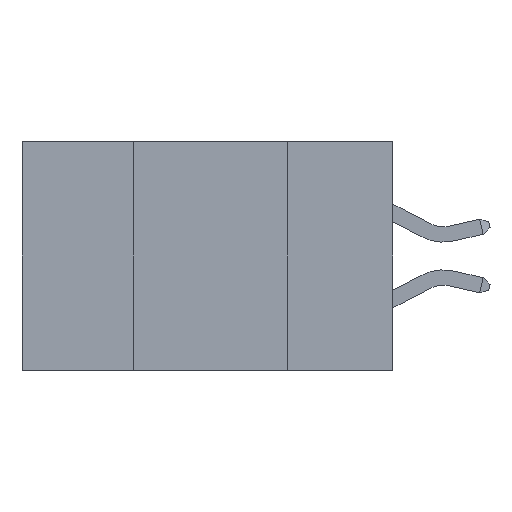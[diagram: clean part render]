
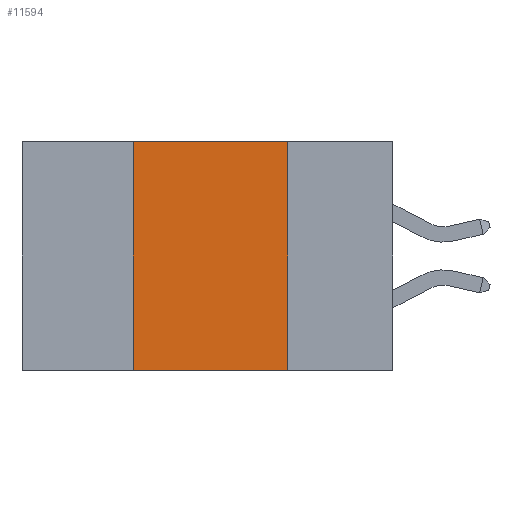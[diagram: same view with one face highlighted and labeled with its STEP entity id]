
A CAD part, left-side view. The second image highlights one B-rep face of the part: STEP entity #11594.
In plain terms, the highlighted planar face has unit normal (-1, 0, 0).
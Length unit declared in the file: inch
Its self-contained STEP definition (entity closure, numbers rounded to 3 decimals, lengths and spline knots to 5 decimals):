
#779 = CARTESIAN_POINT ( 'NONE',  ( 0., 0.6, -0.37 ) ) ;
#1283 = EDGE_CURVE ( 'NONE', #11097, #8057, #9412, .T. ) ;
#1348 = CARTESIAN_POINT ( 'NONE',  ( 0., 0.17, -0.37 ) ) ;
#2622 = DIRECTION ( 'NONE',  ( 0., -1., 0. ) ) ;
#2745 = CARTESIAN_POINT ( 'NONE',  ( 0., 0.6, 0. ) ) ;
#2826 = DIRECTION ( 'NONE',  ( 1., 0., 0. ) ) ;
#4833 = DIRECTION ( 'NONE',  ( 0., 0., 1. ) ) ;
#6314 = EDGE_CURVE ( 'NONE', #17043, #8785, #16749, .T. ) ;
#8057 = VERTEX_POINT ( 'NONE', #10679 ) ;
#8785 = VERTEX_POINT ( 'NONE', #1348 ) ;
#9412 = LINE ( 'NONE', #17453, #14383 ) ;
#9676 = FACE_OUTER_BOUND ( 'NONE', #22063, .T. ) ;
#10679 = CARTESIAN_POINT ( 'NONE',  ( 0., 0.42, 0. ) ) ;
#10813 = CARTESIAN_POINT ( 'NONE',  ( 0., 0.42, -0.37 ) ) ;
#11097 = VERTEX_POINT ( 'NONE', #10813 ) ;
#11594 = ADVANCED_FACE ( 'NONE', ( #9676 ), #14069, .F. ) ;
#11792 = VECTOR ( 'NONE', #14013, 39.37008 ) ;
#12068 = EDGE_CURVE ( 'NONE', #8057, #17043, #14042, .T. ) ;
#14013 = DIRECTION ( 'NONE',  ( 0., 0., -1. ) ) ;
#14042 = LINE ( 'NONE', #15664, #23804 ) ;
#14069 = PLANE ( 'NONE',  #20778 ) ;
#14220 = CARTESIAN_POINT ( 'NONE',  ( 0., 0.17, 0. ) ) ;
#14383 = VECTOR ( 'NONE', #4833, 39.37008 ) ;
#14479 = LINE ( 'NONE', #779, #15062 ) ;
#15062 = VECTOR ( 'NONE', #2622, 39.37008 ) ;
#15515 = ORIENTED_EDGE ( 'NONE', *, *, #6314, .F. ) ;
#15566 = EDGE_CURVE ( 'NONE', #11097, #8785, #14479, .T. ) ;
#15664 = CARTESIAN_POINT ( 'NONE',  ( 0., 0.6, 0. ) ) ;
#15783 = ORIENTED_EDGE ( 'NONE', *, *, #12068, .F. ) ;
#15835 = ORIENTED_EDGE ( 'NONE', *, *, #1283, .F. ) ;
#15853 = ORIENTED_EDGE ( 'NONE', *, *, #15566, .T. ) ;
#15883 = CARTESIAN_POINT ( 'NONE',  ( 0., 0.17, 0. ) ) ;
#15944 = DIRECTION ( 'NONE',  ( 0., 0., -1. ) ) ;
#16749 = LINE ( 'NONE', #15883, #11792 ) ;
#17043 = VERTEX_POINT ( 'NONE', #14220 ) ;
#17453 = CARTESIAN_POINT ( 'NONE',  ( 0., 0.42, 0. ) ) ;
#17548 = DIRECTION ( 'NONE',  ( 0., -1., 0. ) ) ;
#20778 = AXIS2_PLACEMENT_3D ( 'NONE', #2745, #2826, #15944 ) ;
#22063 = EDGE_LOOP ( 'NONE', ( #15515, #15783, #15835, #15853 ) ) ;
#23804 = VECTOR ( 'NONE', #17548, 39.37008 ) ;
